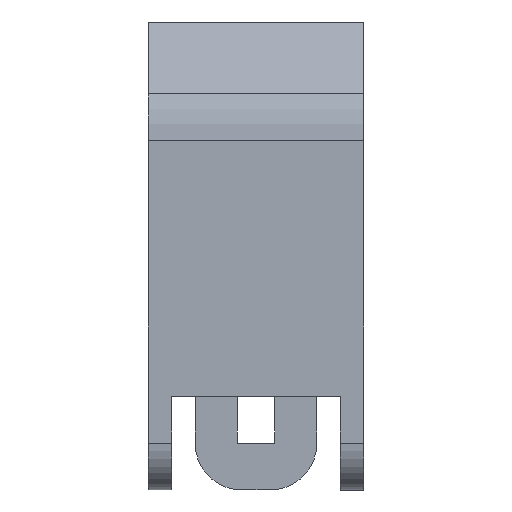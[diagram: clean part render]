
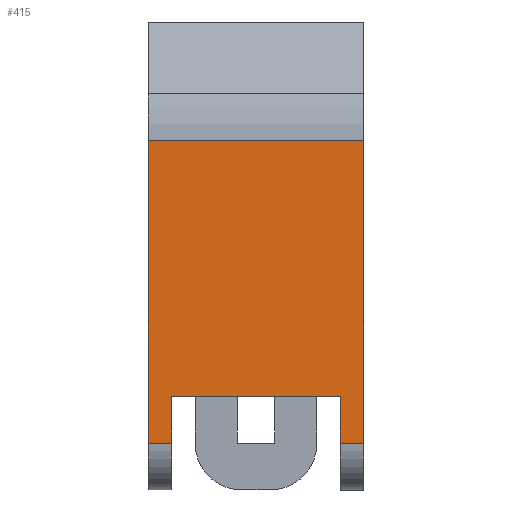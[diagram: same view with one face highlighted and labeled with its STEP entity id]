
A CAD part, front view. The second image highlights one B-rep face of the part: STEP entity #415.
In plain terms, the highlighted planar face has unit normal (0, -1, 0).
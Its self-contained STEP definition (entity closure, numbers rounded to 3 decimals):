
#115 = VERTEX_POINT ( 'NONE', #4796 ) ;
#122 = ORIENTED_EDGE ( 'NONE', *, *, #2414, .F. ) ;
#221 = CARTESIAN_POINT ( 'NONE',  ( 9., -17.5, -5. ) ) ;
#415 = ADVANCED_FACE ( 'NONE', ( #441 ), #7384, .F. ) ;
#441 = FACE_OUTER_BOUND ( 'NONE', #3114, .T. ) ;
#890 = VERTEX_POINT ( 'NONE', #3181 ) ;
#917 = ORIENTED_EDGE ( 'NONE', *, *, #4431, .T. ) ;
#924 = VECTOR ( 'NONE', #5120, 1000. ) ;
#1032 = CARTESIAN_POINT ( 'NONE',  ( -11.5, -17.5, 27.321 ) ) ;
#1518 = VECTOR ( 'NONE', #9779, 1000. ) ;
#1641 = EDGE_CURVE ( 'NONE', #10147, #890, #10806, .T. ) ;
#1751 = AXIS2_PLACEMENT_3D ( 'NONE', #4082, #10865, #5794 ) ;
#1860 = VERTEX_POINT ( 'NONE', #8361 ) ;
#1861 = DIRECTION ( 'NONE',  ( -1., 0., 0. ) ) ;
#2204 = ORIENTED_EDGE ( 'NONE', *, *, #1641, .F. ) ;
#2353 = VECTOR ( 'NONE', #10273, 1000. ) ;
#2414 = EDGE_CURVE ( 'NONE', #115, #2607, #2683, .T. ) ;
#2559 = CARTESIAN_POINT ( 'NONE',  ( -9., -17.5, 40. ) ) ;
#2607 = VERTEX_POINT ( 'NONE', #221 ) ;
#2683 = LINE ( 'NONE', #5032, #6949 ) ;
#2887 = ORIENTED_EDGE ( 'NONE', *, *, #6781, .F. ) ;
#2997 = CARTESIAN_POINT ( 'NONE',  ( -11.5, -17.5, 40. ) ) ;
#3114 = EDGE_LOOP ( 'NONE', ( #2887, #8602, #2204, #9787, #6318, #3742, #917, #122 ) ) ;
#3181 = CARTESIAN_POINT ( 'NONE',  ( -11.5, -17.5, 27.321 ) ) ;
#3367 = VERTEX_POINT ( 'NONE', #6264 ) ;
#3391 = DIRECTION ( 'NONE',  ( 0., 0., 1. ) ) ;
#3742 = ORIENTED_EDGE ( 'NONE', *, *, #4371, .T. ) ;
#4076 = CARTESIAN_POINT ( 'NONE',  ( -9., -17.5, -5. ) ) ;
#4082 = CARTESIAN_POINT ( 'NONE',  ( 9., -17.5, 40. ) ) ;
#4095 = VECTOR ( 'NONE', #1861, 1000. ) ;
#4282 = CARTESIAN_POINT ( 'NONE',  ( -11.5, -17.5, -5. ) ) ;
#4303 = CARTESIAN_POINT ( 'NONE',  ( 9., -17.5, 0. ) ) ;
#4371 = EDGE_CURVE ( 'NONE', #3367, #10227, #10470, .T. ) ;
#4373 = LINE ( 'NONE', #1032, #4095 ) ;
#4431 = EDGE_CURVE ( 'NONE', #10227, #2607, #9151, .T. ) ;
#4501 = EDGE_CURVE ( 'NONE', #1860, #890, #4373, .T. ) ;
#4681 = VECTOR ( 'NONE', #7538, 1000. ) ;
#4796 = CARTESIAN_POINT ( 'NONE',  ( 11.5, -17.5, -5. ) ) ;
#5016 = CARTESIAN_POINT ( 'NONE',  ( 9., -17.5, 0. ) ) ;
#5032 = CARTESIAN_POINT ( 'NONE',  ( 11.5, -17.5, -5. ) ) ;
#5120 = DIRECTION ( 'NONE',  ( 1., 0., 0. ) ) ;
#5166 = DIRECTION ( 'NONE',  ( 1., 0., 0. ) ) ;
#5794 = DIRECTION ( 'NONE',  ( -1., 0., 0. ) ) ;
#6040 = CARTESIAN_POINT ( 'NONE',  ( 9., -17.5, -5. ) ) ;
#6264 = CARTESIAN_POINT ( 'NONE',  ( -9., -17.5, 0. ) ) ;
#6318 = ORIENTED_EDGE ( 'NONE', *, *, #7557, .T. ) ;
#6781 = EDGE_CURVE ( 'NONE', #1860, #115, #9204, .T. ) ;
#6949 = VECTOR ( 'NONE', #10961, 1000. ) ;
#7383 = VECTOR ( 'NONE', #3391, 1000. ) ;
#7384 = PLANE ( 'NONE',  #1751 ) ;
#7538 = DIRECTION ( 'NONE',  ( 0., 0., -1. ) ) ;
#7557 = EDGE_CURVE ( 'NONE', #10171, #3367, #9658, .T. ) ;
#8361 = CARTESIAN_POINT ( 'NONE',  ( 11.5, -17.5, 27.321 ) ) ;
#8389 = CARTESIAN_POINT ( 'NONE',  ( 11.5, -17.5, -5. ) ) ;
#8593 = VECTOR ( 'NONE', #5166, 1000. ) ;
#8602 = ORIENTED_EDGE ( 'NONE', *, *, #4501, .T. ) ;
#9151 = LINE ( 'NONE', #6040, #2353 ) ;
#9204 = LINE ( 'NONE', #8389, #4681 ) ;
#9658 = LINE ( 'NONE', #2559, #7383 ) ;
#9779 = DIRECTION ( 'NONE',  ( 0., 0., 1. ) ) ;
#9787 = ORIENTED_EDGE ( 'NONE', *, *, #9835, .T. ) ;
#9835 = EDGE_CURVE ( 'NONE', #10147, #10171, #10829, .T. ) ;
#10147 = VERTEX_POINT ( 'NONE', #10857 ) ;
#10171 = VERTEX_POINT ( 'NONE', #4076 ) ;
#10227 = VERTEX_POINT ( 'NONE', #5016 ) ;
#10273 = DIRECTION ( 'NONE',  ( 0., 0., -1. ) ) ;
#10470 = LINE ( 'NONE', #4303, #924 ) ;
#10806 = LINE ( 'NONE', #2997, #1518 ) ;
#10829 = LINE ( 'NONE', #4282, #8593 ) ;
#10857 = CARTESIAN_POINT ( 'NONE',  ( -11.5, -17.5, -5. ) ) ;
#10865 = DIRECTION ( 'NONE',  ( 0., 1., 0. ) ) ;
#10961 = DIRECTION ( 'NONE',  ( -1., 0., 0. ) ) ;
